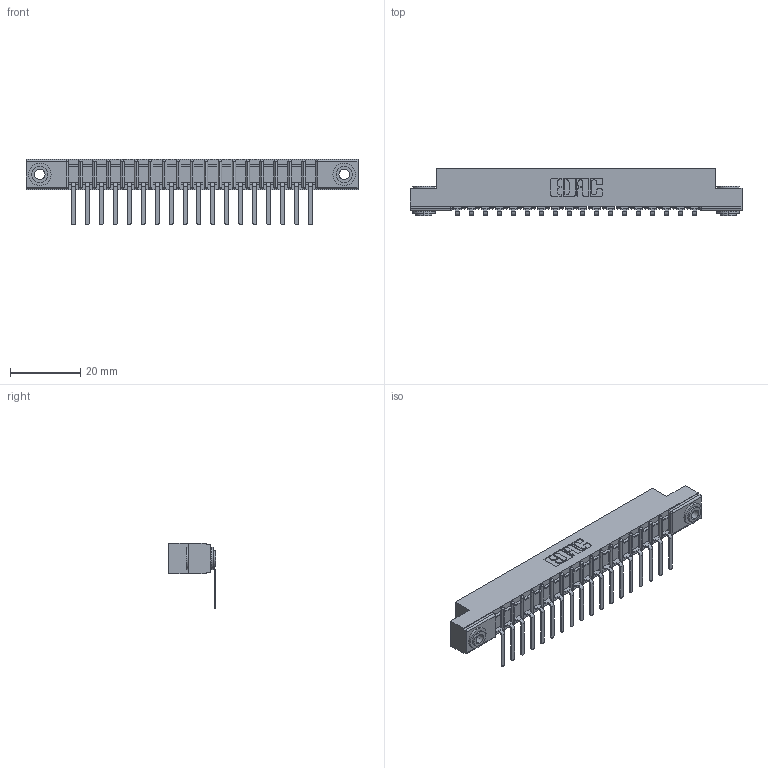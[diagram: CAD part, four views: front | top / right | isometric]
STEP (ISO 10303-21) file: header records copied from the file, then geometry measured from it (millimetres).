
FILE_DESCRIPTION (( 'STEP AP203' ), '1' );
FILE_NAME ('307-018-457-103.STEP', '2020-09-26T01:00:09', ( '' ), ( '' ), 'SwSTEP 2.0', 'SolidWorks 2020', '' );
FILE_SCHEMA (( 'CONFIG_CONTROL_DESIGN' ));
Length unit declared in the file: inch
Products named in the file (4): 307 Part_.156 Dia Mounting Holes; 307-018-457-103; 307-290-002_557; 345-250-002_345-250-002-102
Assembly tree (21 placements, depth 2):
  307-018-457-103
    307 Part_.156 Dia Mounting Holes
    307-290-002_557  x18
    345-250-002_345-250-002-102  x2
Bounding box: 94.34 x 13.36 x 18.67 mm (x, y, z)
Volume: 6275.6 mm3; surface area: 11732.7 mm2
Topology: 21 solids, 21 shells, 1593 faces, 4827 edges, 3162 vertices
Faces by surface type: plane 940, cylinder 607, sphere 38, cone 8
Entity records: 20309 total; most frequent: CARTESIAN_POINT 3401, ORIENTED_EDGE 3382, DIRECTION 3331, EDGE_CURVE 1691, LINE 1275, VECTOR 1275, VERTEX_POINT 1098, AXIS2_PLACEMENT_3D 1028
